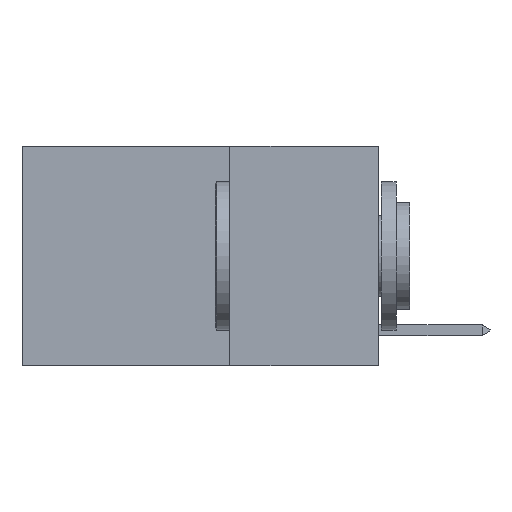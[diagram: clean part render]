
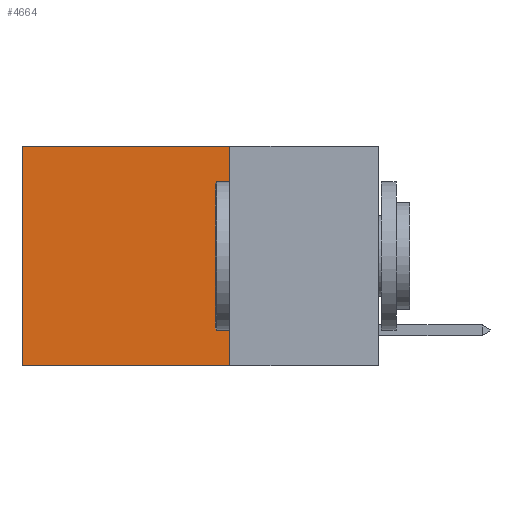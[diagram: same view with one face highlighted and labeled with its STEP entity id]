
A CAD part, left-side view. The second image highlights one B-rep face of the part: STEP entity #4664.
In plain terms, the highlighted planar face has unit normal (-1, 0, 0).
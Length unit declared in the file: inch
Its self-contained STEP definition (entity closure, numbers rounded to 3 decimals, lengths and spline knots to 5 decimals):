
#124 = CARTESIAN_POINT ( 'NONE',  ( 0.2625, 0.25, -0.37 ) ) ;
#486 = VERTEX_POINT ( 'NONE', #8054 ) ;
#1575 = LINE ( 'NONE', #3358, #5390 ) ;
#1685 = CARTESIAN_POINT ( 'NONE',  ( 0.2625, 0.6, -0.37 ) ) ;
#1861 = EDGE_CURVE ( 'NONE', #9397, #5425, #3252, .T. ) ;
#1980 = CARTESIAN_POINT ( 'NONE',  ( 0.2625, 0.25, 0. ) ) ;
#2725 = FACE_OUTER_BOUND ( 'NONE', #4345, .T. ) ;
#2827 = VECTOR ( 'NONE', #8426, 39.37008 ) ;
#2894 = CARTESIAN_POINT ( 'NONE',  ( 0.2625, 0.6, 0. ) ) ;
#3252 = LINE ( 'NONE', #4831, #10157 ) ;
#3349 = LINE ( 'NONE', #124, #3921 ) ;
#3358 = CARTESIAN_POINT ( 'NONE',  ( 0.2625, 0.25, 0. ) ) ;
#3380 = AXIS2_PLACEMENT_3D ( 'NONE', #1980, #8999, #3502 ) ;
#3502 = DIRECTION ( 'NONE',  ( 0., 0., -1. ) ) ;
#3921 = VECTOR ( 'NONE', #8733, 39.37008 ) ;
#4100 = DIRECTION ( 'NONE',  ( 0., 0., -1. ) ) ;
#4345 = EDGE_LOOP ( 'NONE', ( #4928, #6278, #8302, #9249 ) ) ;
#4368 = CARTESIAN_POINT ( 'NONE',  ( 0.2625, 0.25, 0. ) ) ;
#4416 = LINE ( 'NONE', #4368, #2827 ) ;
#4664 = ADVANCED_FACE ( 'NONE', ( #2725 ), #7459, .F. ) ;
#4831 = CARTESIAN_POINT ( 'NONE',  ( 0.2625, 0.6, 0. ) ) ;
#4928 = ORIENTED_EDGE ( 'NONE', *, *, #1861, .T. ) ;
#5390 = VECTOR ( 'NONE', #8895, 39.37008 ) ;
#5425 = VERTEX_POINT ( 'NONE', #1685 ) ;
#5784 = EDGE_CURVE ( 'NONE', #486, #6662, #1575, .T. ) ;
#6242 = EDGE_CURVE ( 'NONE', #6662, #5425, #3349, .T. ) ;
#6278 = ORIENTED_EDGE ( 'NONE', *, *, #6242, .F. ) ;
#6662 = VERTEX_POINT ( 'NONE', #9407 ) ;
#7459 = PLANE ( 'NONE',  #3380 ) ;
#8054 = CARTESIAN_POINT ( 'NONE',  ( 0.2625, 0.25, 0. ) ) ;
#8302 = ORIENTED_EDGE ( 'NONE', *, *, #5784, .F. ) ;
#8426 = DIRECTION ( 'NONE',  ( 0., 1., 0. ) ) ;
#8733 = DIRECTION ( 'NONE',  ( 0., 1., 0. ) ) ;
#8895 = DIRECTION ( 'NONE',  ( 0., 0., -1. ) ) ;
#8999 = DIRECTION ( 'NONE',  ( 1., 0., 0. ) ) ;
#9249 = ORIENTED_EDGE ( 'NONE', *, *, #9349, .T. ) ;
#9349 = EDGE_CURVE ( 'NONE', #486, #9397, #4416, .T. ) ;
#9397 = VERTEX_POINT ( 'NONE', #2894 ) ;
#9407 = CARTESIAN_POINT ( 'NONE',  ( 0.2625, 0.25, -0.37 ) ) ;
#10157 = VECTOR ( 'NONE', #4100, 39.37008 ) ;
